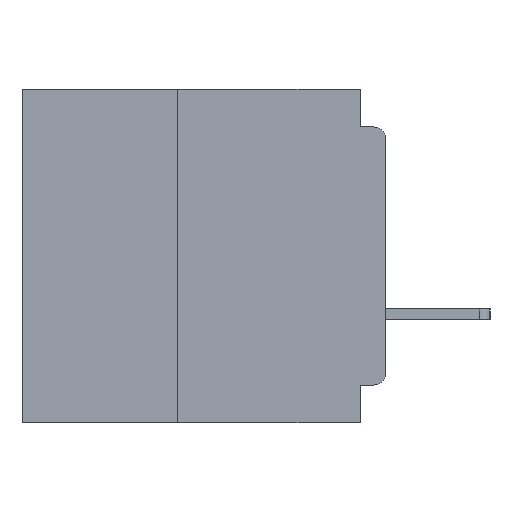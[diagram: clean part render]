
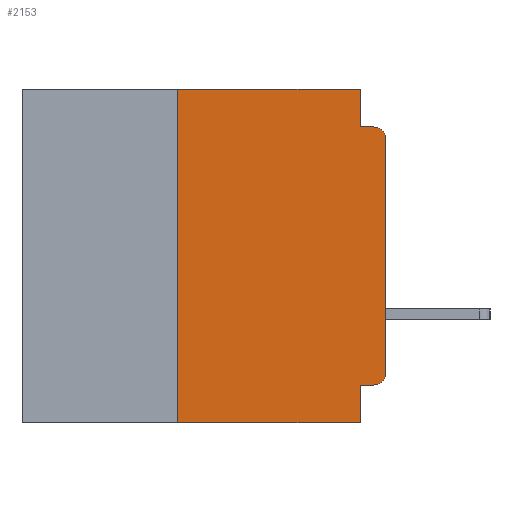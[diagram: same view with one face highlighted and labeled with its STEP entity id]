
A CAD part, left-side view. The second image highlights one B-rep face of the part: STEP entity #2153.
In plain terms, the highlighted planar face has unit normal (-1, 0, 0).
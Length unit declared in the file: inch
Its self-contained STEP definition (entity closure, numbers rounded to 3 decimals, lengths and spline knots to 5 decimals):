
#383 = VERTEX_POINT ( 'NONE', #21662 ) ;
#1215 = CARTESIAN_POINT ( 'NONE',  ( 0., 0.031, 0. ) ) ;
#1799 = EDGE_CURVE ( 'NONE', #14390, #19969, #52594, .T. ) ;
#2153 = ADVANCED_FACE ( 'NONE', ( #43491 ), #30392, .F. ) ;
#3266 = DIRECTION ( 'NONE',  ( 0., 0., -1. ) ) ;
#4232 = DIRECTION ( 'NONE',  ( 0., 0., -1. ) ) ;
#4385 = EDGE_CURVE ( 'NONE', #55614, #65687, #50588, .T. ) ;
#4998 = DIRECTION ( 'NONE',  ( 0., 0., -1. ) ) ;
#5188 = ORIENTED_EDGE ( 'NONE', *, *, #1799, .T. ) ;
#5204 = LINE ( 'NONE', #55991, #12659 ) ;
#5244 = LINE ( 'NONE', #56808, #45864 ) ;
#5539 = DIRECTION ( 'NONE',  ( -1., 0., 0. ) ) ;
#5911 = CARTESIAN_POINT ( 'NONE',  ( 0., 0.437, -0.4 ) ) ;
#5915 = CARTESIAN_POINT ( 'NONE',  ( 0., 0.015, -0.34 ) ) ;
#6652 = EDGE_CURVE ( 'NONE', #24870, #38062, #9502, .T. ) ;
#7166 = VECTOR ( 'NONE', #67837, 39.37008 ) ;
#7436 = ORIENTED_EDGE ( 'NONE', *, *, #24972, .F. ) ;
#8356 = DIRECTION ( 'NONE',  ( 0., 1., 0. ) ) ;
#9502 = LINE ( 'NONE', #45492, #51709 ) ;
#9510 = VECTOR ( 'NONE', #36743, 39.37008 ) ;
#9557 = CARTESIAN_POINT ( 'NONE',  ( 0., 0.25, -0.4 ) ) ;
#11133 = AXIS2_PLACEMENT_3D ( 'NONE', #66725, #34977, #3266 ) ;
#11159 = LINE ( 'NONE', #17939, #50092 ) ;
#12564 = CARTESIAN_POINT ( 'NONE',  ( 0., 0.015, -0.355 ) ) ;
#12659 = VECTOR ( 'NONE', #8356, 39.37008 ) ;
#13547 = LINE ( 'NONE', #5911, #54117 ) ;
#14390 = VERTEX_POINT ( 'NONE', #12564 ) ;
#14518 = CARTESIAN_POINT ( 'NONE',  ( 0., 0., -0.34 ) ) ;
#14666 = ORIENTED_EDGE ( 'NONE', *, *, #66847, .T. ) ;
#16002 = ORIENTED_EDGE ( 'NONE', *, *, #4385, .T. ) ;
#16217 = ORIENTED_EDGE ( 'NONE', *, *, #27343, .F. ) ;
#17939 = CARTESIAN_POINT ( 'NONE',  ( 0., 0., 0. ) ) ;
#17973 = LINE ( 'NONE', #27273, #44505 ) ;
#19084 = DIRECTION ( 'NONE',  ( 0., 0., -1. ) ) ;
#19969 = VERTEX_POINT ( 'NONE', #14518 ) ;
#21662 = CARTESIAN_POINT ( 'NONE',  ( 0., 0.25, 0. ) ) ;
#21668 = AXIS2_PLACEMENT_3D ( 'NONE', #62342, #35974, #4232 ) ;
#23583 = ORIENTED_EDGE ( 'NONE', *, *, #43616, .T. ) ;
#23596 = LINE ( 'NONE', #26090, #9510 ) ;
#23807 = ORIENTED_EDGE ( 'NONE', *, *, #61741, .F. ) ;
#24770 = CARTESIAN_POINT ( 'NONE',  ( 0., 0.031, -0.355 ) ) ;
#24870 = VERTEX_POINT ( 'NONE', #24770 ) ;
#24972 = EDGE_CURVE ( 'NONE', #48972, #383, #63527, .T. ) ;
#25742 = ORIENTED_EDGE ( 'NONE', *, *, #6652, .F. ) ;
#26090 = CARTESIAN_POINT ( 'NONE',  ( 0., 0.437, 0. ) ) ;
#27273 = CARTESIAN_POINT ( 'NONE',  ( 0., 0., -0.045 ) ) ;
#27343 = EDGE_CURVE ( 'NONE', #32004, #59752, #5244, .T. ) ;
#30392 = PLANE ( 'NONE',  #21668 ) ;
#30436 = DIRECTION ( 'NONE',  ( 0., 0., -1. ) ) ;
#31267 = EDGE_CURVE ( 'NONE', #383, #32004, #23596, .T. ) ;
#32004 = VERTEX_POINT ( 'NONE', #1215 ) ;
#32603 = DIRECTION ( 'NONE',  ( 0., -1., 0. ) ) ;
#34948 = AXIS2_PLACEMENT_3D ( 'NONE', #5915, #5539, #4998 ) ;
#34977 = DIRECTION ( 'NONE',  ( -1., 0., 0. ) ) ;
#35974 = DIRECTION ( 'NONE',  ( 1., 0., 0. ) ) ;
#36743 = DIRECTION ( 'NONE',  ( 0., -1., 0. ) ) ;
#38062 = VERTEX_POINT ( 'NONE', #61643 ) ;
#39032 = DIRECTION ( 'NONE',  ( 0., 0., 1. ) ) ;
#40320 = EDGE_LOOP ( 'NONE', ( #23583, #16002, #23807, #16217, #59094, #7436, #14666, #25742, #50854, #5188 ) ) ;
#41420 = CARTESIAN_POINT ( 'NONE',  ( 0., 0.25, -0.4 ) ) ;
#43491 = FACE_OUTER_BOUND ( 'NONE', #40320, .T. ) ;
#43616 = EDGE_CURVE ( 'NONE', #19969, #55614, #11159, .T. ) ;
#44377 = EDGE_CURVE ( 'NONE', #14390, #24870, #5204, .T. ) ;
#44505 = VECTOR ( 'NONE', #32603, 39.37008 ) ;
#45492 = CARTESIAN_POINT ( 'NONE',  ( 0., 0.031, -0.4 ) ) ;
#45864 = VECTOR ( 'NONE', #30436, 39.37008 ) ;
#48932 = CARTESIAN_POINT ( 'NONE',  ( 0., 0.015, -0.045 ) ) ;
#48972 = VERTEX_POINT ( 'NONE', #9557 ) ;
#50092 = VECTOR ( 'NONE', #39032, 39.37008 ) ;
#50588 = CIRCLE ( 'NONE', #11133, 0.015 ) ;
#50854 = ORIENTED_EDGE ( 'NONE', *, *, #44377, .F. ) ;
#51709 = VECTOR ( 'NONE', #19084, 39.37008 ) ;
#52594 = CIRCLE ( 'NONE', #34948, 0.015 ) ;
#54117 = VECTOR ( 'NONE', #58678, 39.37008 ) ;
#55614 = VERTEX_POINT ( 'NONE', #57167 ) ;
#55991 = CARTESIAN_POINT ( 'NONE',  ( 0., 0., -0.355 ) ) ;
#56808 = CARTESIAN_POINT ( 'NONE',  ( 0., 0.031, 0. ) ) ;
#57167 = CARTESIAN_POINT ( 'NONE',  ( 0., 0., -0.06 ) ) ;
#58678 = DIRECTION ( 'NONE',  ( 0., -1., 0. ) ) ;
#59094 = ORIENTED_EDGE ( 'NONE', *, *, #31267, .F. ) ;
#59752 = VERTEX_POINT ( 'NONE', #62197 ) ;
#61643 = CARTESIAN_POINT ( 'NONE',  ( 0., 0.031, -0.4 ) ) ;
#61741 = EDGE_CURVE ( 'NONE', #59752, #65687, #17973, .T. ) ;
#62197 = CARTESIAN_POINT ( 'NONE',  ( 0., 0.031, -0.045 ) ) ;
#62342 = CARTESIAN_POINT ( 'NONE',  ( 0., 0.437, 0. ) ) ;
#63527 = LINE ( 'NONE', #41420, #7166 ) ;
#65687 = VERTEX_POINT ( 'NONE', #48932 ) ;
#66725 = CARTESIAN_POINT ( 'NONE',  ( 0., 0.015, -0.06 ) ) ;
#66847 = EDGE_CURVE ( 'NONE', #48972, #38062, #13547, .T. ) ;
#67837 = DIRECTION ( 'NONE',  ( 0., 0., 1. ) ) ;
